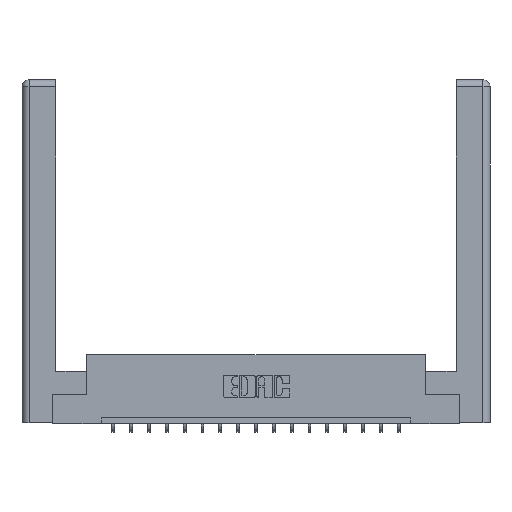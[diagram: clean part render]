
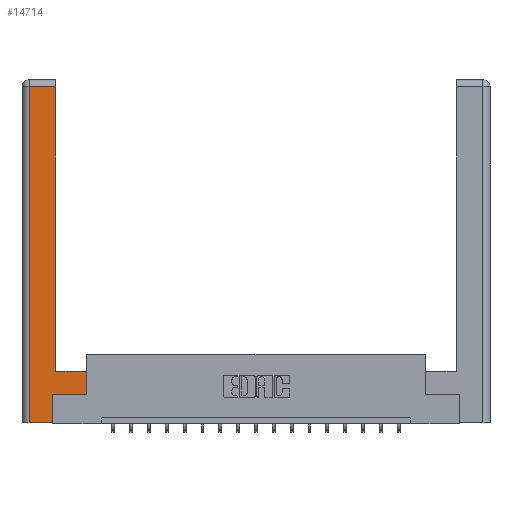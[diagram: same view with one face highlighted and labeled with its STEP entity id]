
A CAD part, top view. The second image highlights one B-rep face of the part: STEP entity #14714.
In plain terms, the highlighted planar face has unit normal (0, 0, 1).
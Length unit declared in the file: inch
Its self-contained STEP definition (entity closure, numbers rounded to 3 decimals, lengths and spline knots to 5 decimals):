
#76 = LINE ( 'NONE', #17899, #6814 ) ;
#1418 = CARTESIAN_POINT ( 'NONE',  ( 0.565, 0.45, 0. ) ) ;
#2032 = CARTESIAN_POINT ( 'NONE',  ( 0.295, 2.94, 0. ) ) ;
#2049 = VECTOR ( 'NONE', #5699, 39.37008 ) ;
#2450 = EDGE_CURVE ( 'NONE', #7747, #11065, #10575, .T. ) ;
#2451 = CARTESIAN_POINT ( 'NONE',  ( 0.0615, 2.94, 0. ) ) ;
#2555 = VERTEX_POINT ( 'NONE', #6011 ) ;
#3145 = VERTEX_POINT ( 'NONE', #10159 ) ;
#3232 = CARTESIAN_POINT ( 'NONE',  ( 0.265, 0.245, 0. ) ) ;
#3574 = DIRECTION ( 'NONE',  ( 0., 1., 0. ) ) ;
#4195 = CARTESIAN_POINT ( 'NONE',  ( 0.565, 0.245, 0. ) ) ;
#4315 = ORIENTED_EDGE ( 'NONE', *, *, #2450, .T. ) ;
#4387 = ORIENTED_EDGE ( 'NONE', *, *, #12932, .T. ) ;
#4411 = CARTESIAN_POINT ( 'NONE',  ( 0.265, 0., 0. ) ) ;
#4856 = AXIS2_PLACEMENT_3D ( 'NONE', #18144, #12367, #9796 ) ;
#5699 = DIRECTION ( 'NONE',  ( -1., 0., 0. ) ) ;
#5779 = CARTESIAN_POINT ( 'NONE',  ( 0.565, 0.245, 0. ) ) ;
#5885 = LINE ( 'NONE', #14329, #2049 ) ;
#5902 = VECTOR ( 'NONE', #15815, 39.37008 ) ;
#5929 = EDGE_LOOP ( 'NONE', ( #16215, #4387, #18583, #7636, #11099, #7651, #4315, #11802 ) ) ;
#5984 = EDGE_CURVE ( 'NONE', #2555, #7747, #17870, .T. ) ;
#6011 = CARTESIAN_POINT ( 'NONE',  ( 0.265, 0.245, 0. ) ) ;
#6393 = DIRECTION ( 'NONE',  ( -1., 0., 0. ) ) ;
#6550 = VERTEX_POINT ( 'NONE', #2451 ) ;
#6814 = VECTOR ( 'NONE', #6393, 39.37008 ) ;
#7033 = DIRECTION ( 'NONE',  ( 1., 0., 0. ) ) ;
#7224 = EDGE_CURVE ( 'NONE', #15546, #7929, #9727, .T. ) ;
#7636 = ORIENTED_EDGE ( 'NONE', *, *, #7224, .T. ) ;
#7651 = ORIENTED_EDGE ( 'NONE', *, *, #5984, .T. ) ;
#7747 = VERTEX_POINT ( 'NONE', #5779 ) ;
#7929 = VERTEX_POINT ( 'NONE', #4411 ) ;
#9088 = CARTESIAN_POINT ( 'NONE',  ( 0.565, 0.45, 0. ) ) ;
#9218 = VECTOR ( 'NONE', #13338, 39.37008 ) ;
#9631 = CARTESIAN_POINT ( 'NONE',  ( 0.0615, 0., 0. ) ) ;
#9700 = DIRECTION ( 'NONE',  ( 0., -1., 0. ) ) ;
#9727 = LINE ( 'NONE', #14687, #5902 ) ;
#9796 = DIRECTION ( 'NONE',  ( -1., 0., 0. ) ) ;
#10061 = VECTOR ( 'NONE', #3574, 39.37008 ) ;
#10159 = CARTESIAN_POINT ( 'NONE',  ( 0.295, 0.45, 0. ) ) ;
#10575 = LINE ( 'NONE', #1418, #16412 ) ;
#11034 = VECTOR ( 'NONE', #9700, 39.37008 ) ;
#11065 = VERTEX_POINT ( 'NONE', #9088 ) ;
#11099 = ORIENTED_EDGE ( 'NONE', *, *, #16432, .T. ) ;
#11802 = ORIENTED_EDGE ( 'NONE', *, *, #15637, .T. ) ;
#12173 = CARTESIAN_POINT ( 'NONE',  ( 0.295, 3., 0. ) ) ;
#12367 = DIRECTION ( 'NONE',  ( 0., 0., -1. ) ) ;
#12932 = EDGE_CURVE ( 'NONE', #15932, #6550, #76, .T. ) ;
#13338 = DIRECTION ( 'NONE',  ( 0., 1., 0. ) ) ;
#14329 = CARTESIAN_POINT ( 'NONE',  ( 0.295, 0.45, 0. ) ) ;
#14687 = CARTESIAN_POINT ( 'NONE',  ( 0.265, 0., 0. ) ) ;
#14714 = ADVANCED_FACE ( 'NONE', ( #16022 ), #15400, .F. ) ;
#15271 = EDGE_CURVE ( 'NONE', #6550, #15546, #16655, .T. ) ;
#15297 = LINE ( 'NONE', #3232, #9218 ) ;
#15400 = PLANE ( 'NONE',  #4856 ) ;
#15546 = VERTEX_POINT ( 'NONE', #16833 ) ;
#15637 = EDGE_CURVE ( 'NONE', #11065, #3145, #5885, .T. ) ;
#15815 = DIRECTION ( 'NONE',  ( 1., 0., 0. ) ) ;
#15932 = VERTEX_POINT ( 'NONE', #2032 ) ;
#16022 = FACE_OUTER_BOUND ( 'NONE', #5929, .T. ) ;
#16215 = ORIENTED_EDGE ( 'NONE', *, *, #18110, .T. ) ;
#16412 = VECTOR ( 'NONE', #17382, 39.37008 ) ;
#16432 = EDGE_CURVE ( 'NONE', #7929, #2555, #15297, .T. ) ;
#16655 = LINE ( 'NONE', #9631, #11034 ) ;
#16833 = CARTESIAN_POINT ( 'NONE',  ( 0.0615, 0., 0. ) ) ;
#17382 = DIRECTION ( 'NONE',  ( 0., 1., 0. ) ) ;
#17432 = VECTOR ( 'NONE', #7033, 39.37008 ) ;
#17685 = LINE ( 'NONE', #12173, #10061 ) ;
#17870 = LINE ( 'NONE', #4195, #17432 ) ;
#17899 = CARTESIAN_POINT ( 'NONE',  ( 0.0615, 2.94, 0. ) ) ;
#18110 = EDGE_CURVE ( 'NONE', #3145, #15932, #17685, .T. ) ;
#18144 = CARTESIAN_POINT ( 'NONE',  ( 0., 0., 0. ) ) ;
#18583 = ORIENTED_EDGE ( 'NONE', *, *, #15271, .T. ) ;
